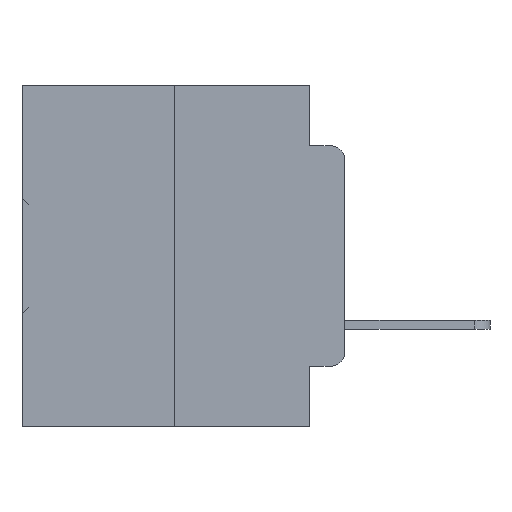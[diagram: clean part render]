
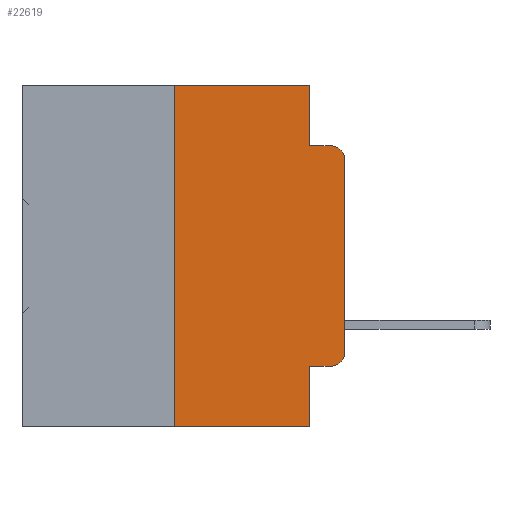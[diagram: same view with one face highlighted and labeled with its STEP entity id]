
A CAD part, left-side view. The second image highlights one B-rep face of the part: STEP entity #22619.
In plain terms, the highlighted planar face has unit normal (-1, 0, 0).
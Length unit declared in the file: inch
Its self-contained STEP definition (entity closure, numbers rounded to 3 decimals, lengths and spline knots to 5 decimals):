
#1632 = ORIENTED_EDGE ( 'NONE', *, *, #12065, .F. ) ;
#1877 = VERTEX_POINT ( 'NONE', #19949 ) ;
#2384 = CARTESIAN_POINT ( 'NONE',  ( 0., 0.473, 0. ) ) ;
#2967 = CARTESIAN_POINT ( 'NONE',  ( 0., 0.051, -0.4115 ) ) ;
#4075 = ORIENTED_EDGE ( 'NONE', *, *, #11911, .T. ) ;
#4180 = VERTEX_POINT ( 'NONE', #17977 ) ;
#4648 = CARTESIAN_POINT ( 'NONE',  ( 0., 0.473, 0. ) ) ;
#5728 = CARTESIAN_POINT ( 'NONE',  ( 0., 0.02, -0.0885 ) ) ;
#6124 = FACE_OUTER_BOUND ( 'NONE', #33786, .T. ) ;
#6274 = DIRECTION ( 'NONE',  ( -1., 0., 0. ) ) ;
#6315 = LINE ( 'NONE', #2384, #7267 ) ;
#7088 = LINE ( 'NONE', #33230, #12205 ) ;
#7267 = VECTOR ( 'NONE', #8477, 39.37008 ) ;
#7474 = VERTEX_POINT ( 'NONE', #19560 ) ;
#7549 = VECTOR ( 'NONE', #32767, 39.37008 ) ;
#7665 = PLANE ( 'NONE',  #15048 ) ;
#8112 = DIRECTION ( 'NONE',  ( 0., 0., 1. ) ) ;
#8477 = DIRECTION ( 'NONE',  ( 0., -1., 0. ) ) ;
#8941 = CARTESIAN_POINT ( 'NONE',  ( 0., 0.02, -0.1085 ) ) ;
#9427 = CIRCLE ( 'NONE', #35734, 0.02 ) ;
#9509 = VECTOR ( 'NONE', #13151, 39.37008 ) ;
#10093 = EDGE_CURVE ( 'NONE', #1877, #11587, #6315, .T. ) ;
#10220 = VERTEX_POINT ( 'NONE', #15280 ) ;
#11298 = EDGE_CURVE ( 'NONE', #15861, #4180, #26356, .T. ) ;
#11587 = VERTEX_POINT ( 'NONE', #29095 ) ;
#11911 = EDGE_CURVE ( 'NONE', #21757, #22585, #7088, .T. ) ;
#11946 = DIRECTION ( 'NONE',  ( 0., 0., -1. ) ) ;
#11960 = EDGE_CURVE ( 'NONE', #22585, #24165, #9427, .T. ) ;
#12011 = EDGE_CURVE ( 'NONE', #13583, #24165, #29890, .T. ) ;
#12016 = EDGE_CURVE ( 'NONE', #11587, #13583, #16330, .T. ) ;
#12020 = EDGE_CURVE ( 'NONE', #15861, #1877, #23836, .T. ) ;
#12065 = EDGE_CURVE ( 'NONE', #7474, #4180, #28326, .T. ) ;
#12077 = EDGE_CURVE ( 'NONE', #7474, #10220, #33317, .T. ) ;
#12127 = EDGE_CURVE ( 'NONE', #10220, #21757, #31782, .T. ) ;
#12205 = VECTOR ( 'NONE', #25669, 39.37008 ) ;
#13049 = ORIENTED_EDGE ( 'NONE', *, *, #12077, .T. ) ;
#13151 = DIRECTION ( 'NONE',  ( 0., -1., 0. ) ) ;
#13362 = CARTESIAN_POINT ( 'NONE',  ( 0., 0., -0.1085 ) ) ;
#13566 = VECTOR ( 'NONE', #14212, 39.37008 ) ;
#13583 = VERTEX_POINT ( 'NONE', #20396 ) ;
#13622 = DIRECTION ( 'NONE',  ( 0., 0., -1. ) ) ;
#14212 = DIRECTION ( 'NONE',  ( 0., 0., -1. ) ) ;
#15048 = AXIS2_PLACEMENT_3D ( 'NONE', #4648, #30030, #13622 ) ;
#15280 = CARTESIAN_POINT ( 'NONE',  ( 0., 0.02, -0.4115 ) ) ;
#15382 = VECTOR ( 'NONE', #8112, 39.37008 ) ;
#15861 = VERTEX_POINT ( 'NONE', #35502 ) ;
#16330 = LINE ( 'NONE', #26109, #7549 ) ;
#16618 = ORIENTED_EDGE ( 'NONE', *, *, #10093, .F. ) ;
#17977 = CARTESIAN_POINT ( 'NONE',  ( 0., 0.051, -0.5 ) ) ;
#19390 = ORIENTED_EDGE ( 'NONE', *, *, #12011, .F. ) ;
#19560 = CARTESIAN_POINT ( 'NONE',  ( 0., 0.051, -0.4115 ) ) ;
#19949 = CARTESIAN_POINT ( 'NONE',  ( 0., 0.25, 0. ) ) ;
#20396 = CARTESIAN_POINT ( 'NONE',  ( 0., 0.051, -0.0885 ) ) ;
#21757 = VERTEX_POINT ( 'NONE', #26694 ) ;
#22585 = VERTEX_POINT ( 'NONE', #13362 ) ;
#22619 = ADVANCED_FACE ( 'NONE', ( #6124 ), #7665, .F. ) ;
#23006 = VECTOR ( 'NONE', #27795, 39.37008 ) ;
#23459 = DIRECTION ( 'NONE',  ( 0., -1., 0. ) ) ;
#23502 = CARTESIAN_POINT ( 'NONE',  ( 0., 0.051, -0.0885 ) ) ;
#23680 = CARTESIAN_POINT ( 'NONE',  ( 0., 0.02, -0.3915 ) ) ;
#23780 = ORIENTED_EDGE ( 'NONE', *, *, #12020, .F. ) ;
#23836 = LINE ( 'NONE', #25281, #15382 ) ;
#24165 = VERTEX_POINT ( 'NONE', #5728 ) ;
#24913 = ORIENTED_EDGE ( 'NONE', *, *, #11960, .T. ) ;
#25144 = AXIS2_PLACEMENT_3D ( 'NONE', #23680, #6274, #26299 ) ;
#25281 = CARTESIAN_POINT ( 'NONE',  ( 0., 0.25, 0. ) ) ;
#25429 = ORIENTED_EDGE ( 'NONE', *, *, #11298, .T. ) ;
#25669 = DIRECTION ( 'NONE',  ( 0., 0., 1. ) ) ;
#26109 = CARTESIAN_POINT ( 'NONE',  ( 0., 0.051, 0. ) ) ;
#26299 = DIRECTION ( 'NONE',  ( 0., 0., -1. ) ) ;
#26356 = LINE ( 'NONE', #34433, #9509 ) ;
#26672 = VECTOR ( 'NONE', #23459, 39.37008 ) ;
#26694 = CARTESIAN_POINT ( 'NONE',  ( 0., 0., -0.3915 ) ) ;
#27795 = DIRECTION ( 'NONE',  ( 0., -1., 0. ) ) ;
#28267 = ORIENTED_EDGE ( 'NONE', *, *, #12016, .F. ) ;
#28326 = LINE ( 'NONE', #32983, #13566 ) ;
#28613 = DIRECTION ( 'NONE',  ( -1., 0., 0. ) ) ;
#29095 = CARTESIAN_POINT ( 'NONE',  ( 0., 0.051, 0. ) ) ;
#29890 = LINE ( 'NONE', #23502, #23006 ) ;
#30030 = DIRECTION ( 'NONE',  ( 1., 0., 0. ) ) ;
#31782 = CIRCLE ( 'NONE', #25144, 0.02 ) ;
#32527 = ORIENTED_EDGE ( 'NONE', *, *, #12127, .T. ) ;
#32767 = DIRECTION ( 'NONE',  ( 0., 0., -1. ) ) ;
#32983 = CARTESIAN_POINT ( 'NONE',  ( 0., 0.051, 0. ) ) ;
#33230 = CARTESIAN_POINT ( 'NONE',  ( 0., 0., 0. ) ) ;
#33317 = LINE ( 'NONE', #2967, #26672 ) ;
#33786 = EDGE_LOOP ( 'NONE', ( #4075, #24913, #19390, #28267, #16618, #23780, #25429, #1632, #13049, #32527 ) ) ;
#34433 = CARTESIAN_POINT ( 'NONE',  ( 0., 0.473, -0.5 ) ) ;
#35502 = CARTESIAN_POINT ( 'NONE',  ( 0., 0.25, -0.5 ) ) ;
#35734 = AXIS2_PLACEMENT_3D ( 'NONE', #8941, #28613, #11946 ) ;
